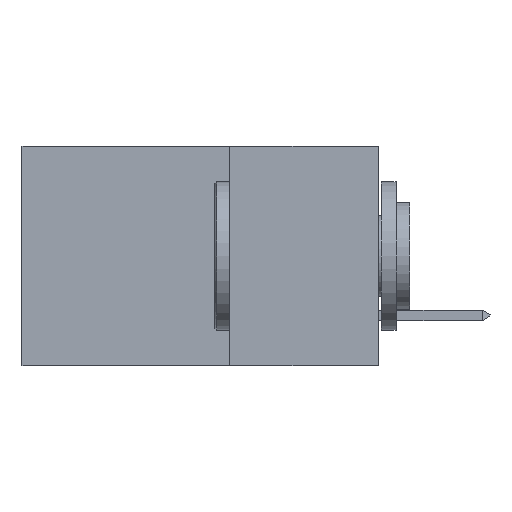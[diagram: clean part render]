
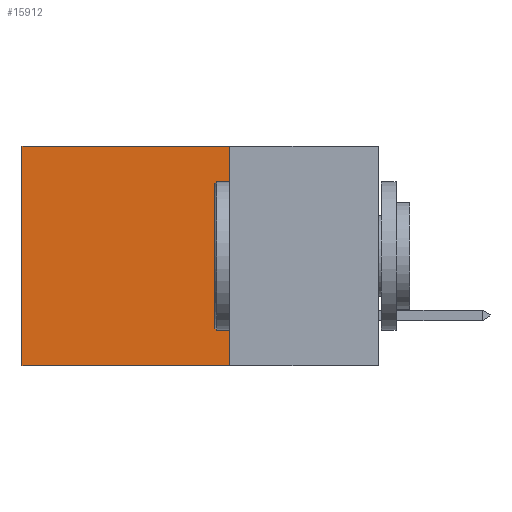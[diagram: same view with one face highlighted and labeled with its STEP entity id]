
A CAD part, left-side view. The second image highlights one B-rep face of the part: STEP entity #15912.
In plain terms, the highlighted planar face has unit normal (-1, 0, 0).
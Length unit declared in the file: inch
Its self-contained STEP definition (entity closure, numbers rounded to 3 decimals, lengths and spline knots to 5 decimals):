
#653 = CARTESIAN_POINT ( 'NONE',  ( 0.298, 0.25, -0.37 ) ) ;
#972 = CARTESIAN_POINT ( 'NONE',  ( 0.298, 0.25, 0. ) ) ;
#1175 = VECTOR ( 'NONE', #4229, 39.37008 ) ;
#2049 = LINE ( 'NONE', #13412, #1175 ) ;
#2268 = VERTEX_POINT ( 'NONE', #10963 ) ;
#3609 = AXIS2_PLACEMENT_3D ( 'NONE', #12594, #14101, #13930 ) ;
#4229 = DIRECTION ( 'NONE',  ( 0., 0., -1. ) ) ;
#4335 = EDGE_CURVE ( 'NONE', #12155, #2268, #5309, .T. ) ;
#5309 = LINE ( 'NONE', #6317, #12803 ) ;
#5363 = LINE ( 'NONE', #14642, #12034 ) ;
#6227 = VECTOR ( 'NONE', #13023, 39.37008 ) ;
#6317 = CARTESIAN_POINT ( 'NONE',  ( 0.298, 0.25, -0.37 ) ) ;
#6506 = ORIENTED_EDGE ( 'NONE', *, *, #16107, .F. ) ;
#6666 = DIRECTION ( 'NONE',  ( 0., 1., 0. ) ) ;
#7468 = ORIENTED_EDGE ( 'NONE', *, *, #11278, .T. ) ;
#9708 = VERTEX_POINT ( 'NONE', #972 ) ;
#10213 = FACE_OUTER_BOUND ( 'NONE', #13421, .T. ) ;
#10707 = ORIENTED_EDGE ( 'NONE', *, *, #4335, .F. ) ;
#10963 = CARTESIAN_POINT ( 'NONE',  ( 0.298, 0.6, -0.37 ) ) ;
#11278 = EDGE_CURVE ( 'NONE', #12209, #2268, #2049, .T. ) ;
#11421 = ORIENTED_EDGE ( 'NONE', *, *, #11836, .T. ) ;
#11836 = EDGE_CURVE ( 'NONE', #9708, #12209, #5363, .T. ) ;
#12034 = VECTOR ( 'NONE', #6666, 39.37008 ) ;
#12155 = VERTEX_POINT ( 'NONE', #653 ) ;
#12209 = VERTEX_POINT ( 'NONE', #13556 ) ;
#12594 = CARTESIAN_POINT ( 'NONE',  ( 0.298, 0.25, 0. ) ) ;
#12774 = PLANE ( 'NONE',  #3609 ) ;
#12803 = VECTOR ( 'NONE', #15606, 39.37008 ) ;
#12966 = CARTESIAN_POINT ( 'NONE',  ( 0.298, 0.25, 0. ) ) ;
#13023 = DIRECTION ( 'NONE',  ( 0., 0., -1. ) ) ;
#13412 = CARTESIAN_POINT ( 'NONE',  ( 0.298, 0.6, 0. ) ) ;
#13421 = EDGE_LOOP ( 'NONE', ( #7468, #10707, #6506, #11421 ) ) ;
#13521 = LINE ( 'NONE', #12966, #6227 ) ;
#13556 = CARTESIAN_POINT ( 'NONE',  ( 0.298, 0.6, 0. ) ) ;
#13930 = DIRECTION ( 'NONE',  ( 0., 0., -1. ) ) ;
#14101 = DIRECTION ( 'NONE',  ( 1., 0., 0. ) ) ;
#14642 = CARTESIAN_POINT ( 'NONE',  ( 0.298, 0.25, 0. ) ) ;
#15606 = DIRECTION ( 'NONE',  ( 0., 1., 0. ) ) ;
#15912 = ADVANCED_FACE ( 'NONE', ( #10213 ), #12774, .F. ) ;
#16107 = EDGE_CURVE ( 'NONE', #9708, #12155, #13521, .T. ) ;
